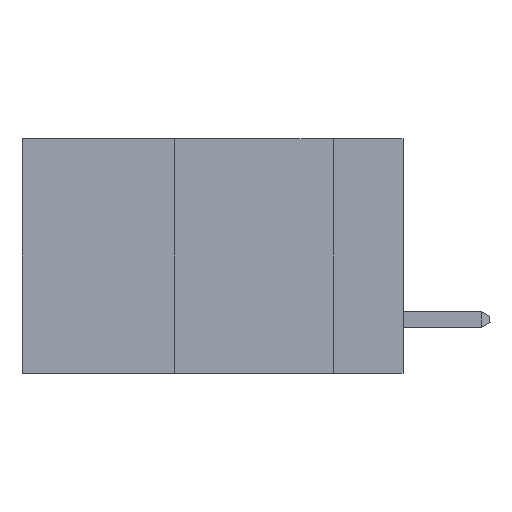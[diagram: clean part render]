
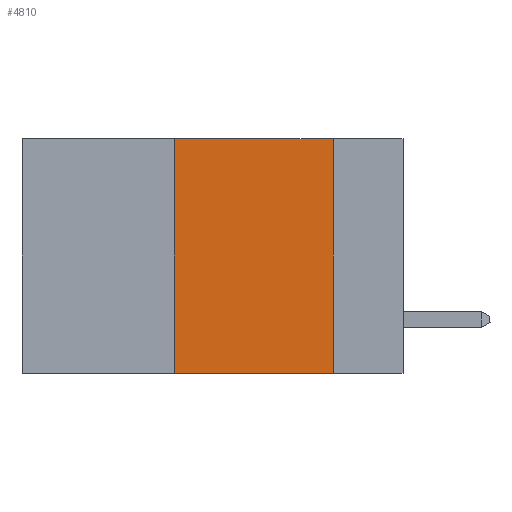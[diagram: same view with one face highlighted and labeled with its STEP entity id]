
A CAD part, left-side view. The second image highlights one B-rep face of the part: STEP entity #4810.
In plain terms, the highlighted planar face has unit normal (-1, 0, 0).
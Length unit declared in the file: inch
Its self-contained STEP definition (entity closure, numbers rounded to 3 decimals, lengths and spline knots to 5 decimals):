
#333 = EDGE_LOOP ( 'NONE', ( #21627, #21726, #22940, #11764 ) ) ;
#473 = CARTESIAN_POINT ( 'NONE',  ( 0., 0.6, 0. ) ) ;
#1249 = VERTEX_POINT ( 'NONE', #11218 ) ;
#2092 = LINE ( 'NONE', #473, #13530 ) ;
#3156 = EDGE_CURVE ( 'NONE', #1249, #6687, #12433, .T. ) ;
#4061 = LINE ( 'NONE', #6036, #12044 ) ;
#4810 = ADVANCED_FACE ( 'NONE', ( #14407 ), #21571, .F. ) ;
#5297 = EDGE_CURVE ( 'NONE', #8058, #13770, #2092, .T. ) ;
#5652 = DIRECTION ( 'NONE',  ( 0., 0., 1. ) ) ;
#5955 = DIRECTION ( 'NONE',  ( 0., 0., -1. ) ) ;
#6036 = CARTESIAN_POINT ( 'NONE',  ( 0., 0.11, 0. ) ) ;
#6687 = VERTEX_POINT ( 'NONE', #20927 ) ;
#8058 = VERTEX_POINT ( 'NONE', #20253 ) ;
#8474 = EDGE_CURVE ( 'NONE', #13770, #6687, #4061, .T. ) ;
#10729 = DIRECTION ( 'NONE',  ( 0., 0., -1. ) ) ;
#10959 = LINE ( 'NONE', #15128, #22715 ) ;
#11218 = CARTESIAN_POINT ( 'NONE',  ( 0., 0.36, -0.37 ) ) ;
#11764 = ORIENTED_EDGE ( 'NONE', *, *, #3156, .T. ) ;
#12044 = VECTOR ( 'NONE', #5955, 39.37008 ) ;
#12433 = LINE ( 'NONE', #13316, #17899 ) ;
#13316 = CARTESIAN_POINT ( 'NONE',  ( 0., 0.6, -0.37 ) ) ;
#13530 = VECTOR ( 'NONE', #18443, 39.37008 ) ;
#13545 = AXIS2_PLACEMENT_3D ( 'NONE', #21714, #18269, #10729 ) ;
#13770 = VERTEX_POINT ( 'NONE', #16190 ) ;
#14407 = FACE_OUTER_BOUND ( 'NONE', #333, .T. ) ;
#15128 = CARTESIAN_POINT ( 'NONE',  ( 0., 0.36, 0. ) ) ;
#16190 = CARTESIAN_POINT ( 'NONE',  ( 0., 0.11, 0. ) ) ;
#17899 = VECTOR ( 'NONE', #18862, 39.37008 ) ;
#18019 = EDGE_CURVE ( 'NONE', #1249, #8058, #10959, .T. ) ;
#18269 = DIRECTION ( 'NONE',  ( 1., 0., 0. ) ) ;
#18443 = DIRECTION ( 'NONE',  ( 0., -1., 0. ) ) ;
#18862 = DIRECTION ( 'NONE',  ( 0., -1., 0. ) ) ;
#20253 = CARTESIAN_POINT ( 'NONE',  ( 0., 0.36, 0. ) ) ;
#20927 = CARTESIAN_POINT ( 'NONE',  ( 0., 0.11, -0.37 ) ) ;
#21571 = PLANE ( 'NONE',  #13545 ) ;
#21627 = ORIENTED_EDGE ( 'NONE', *, *, #8474, .F. ) ;
#21714 = CARTESIAN_POINT ( 'NONE',  ( 0., 0.6, 0. ) ) ;
#21726 = ORIENTED_EDGE ( 'NONE', *, *, #5297, .F. ) ;
#22715 = VECTOR ( 'NONE', #5652, 39.37008 ) ;
#22940 = ORIENTED_EDGE ( 'NONE', *, *, #18019, .F. ) ;
